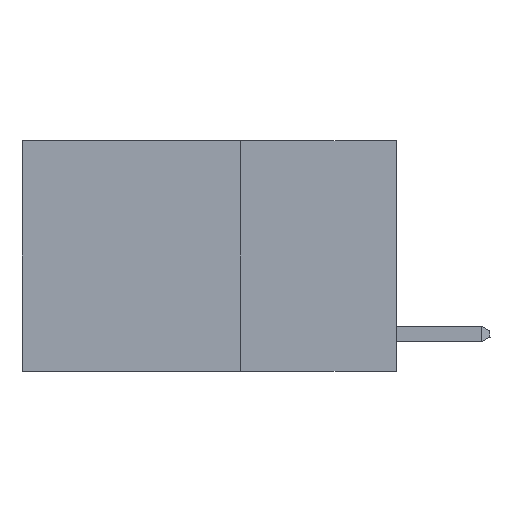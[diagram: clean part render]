
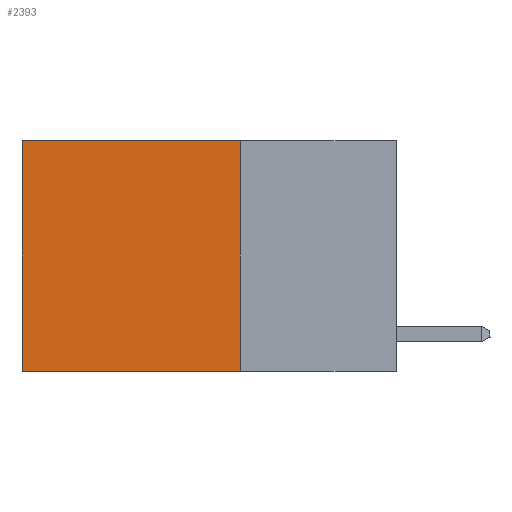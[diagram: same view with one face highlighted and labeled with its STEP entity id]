
A CAD part, left-side view. The second image highlights one B-rep face of the part: STEP entity #2393.
In plain terms, the highlighted planar face has unit normal (-1, 0, 0).
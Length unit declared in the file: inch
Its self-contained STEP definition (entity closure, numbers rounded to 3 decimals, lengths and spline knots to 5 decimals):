
#414 = EDGE_CURVE ( 'NONE', #20700, #18287, #15622, .T. ) ;
#497 = CARTESIAN_POINT ( 'NONE',  ( 0.2625, 0.25, 0. ) ) ;
#1121 = AXIS2_PLACEMENT_3D ( 'NONE', #14091, #20142, #8088 ) ;
#1443 = VERTEX_POINT ( 'NONE', #497 ) ;
#1730 = DIRECTION ( 'NONE',  ( 0., 1., 0. ) ) ;
#2393 = ADVANCED_FACE ( 'NONE', ( #16358 ), #6029, .F. ) ;
#3197 = ORIENTED_EDGE ( 'NONE', *, *, #414, .F. ) ;
#3429 = LINE ( 'NONE', #11577, #14179 ) ;
#4491 = EDGE_LOOP ( 'NONE', ( #7459, #3197, #17044, #9672 ) ) ;
#4577 = VECTOR ( 'NONE', #13738, 39.37008 ) ;
#4591 = CARTESIAN_POINT ( 'NONE',  ( 0.2625, 0.6, -0.37 ) ) ;
#6029 = PLANE ( 'NONE',  #1121 ) ;
#7459 = ORIENTED_EDGE ( 'NONE', *, *, #25188, .T. ) ;
#8088 = DIRECTION ( 'NONE',  ( 0., 0., -1. ) ) ;
#8671 = LINE ( 'NONE', #24523, #13416 ) ;
#9672 = ORIENTED_EDGE ( 'NONE', *, *, #16811, .T. ) ;
#11577 = CARTESIAN_POINT ( 'NONE',  ( 0.2625, 0.25, 0. ) ) ;
#12103 = CARTESIAN_POINT ( 'NONE',  ( 0.2625, 0.6, 0. ) ) ;
#13416 = VECTOR ( 'NONE', #14526, 39.37008 ) ;
#13738 = DIRECTION ( 'NONE',  ( 0., 0., -1. ) ) ;
#14091 = CARTESIAN_POINT ( 'NONE',  ( 0.2625, 0.25, 0. ) ) ;
#14179 = VECTOR ( 'NONE', #25609, 39.37008 ) ;
#14526 = DIRECTION ( 'NONE',  ( 0., 1., 0. ) ) ;
#15622 = LINE ( 'NONE', #21803, #20937 ) ;
#16064 = VERTEX_POINT ( 'NONE', #12103 ) ;
#16358 = FACE_OUTER_BOUND ( 'NONE', #4491, .T. ) ;
#16786 = CARTESIAN_POINT ( 'NONE',  ( 0.2625, 0.25, -0.37 ) ) ;
#16811 = EDGE_CURVE ( 'NONE', #1443, #16064, #8671, .T. ) ;
#17044 = ORIENTED_EDGE ( 'NONE', *, *, #23510, .F. ) ;
#18287 = VERTEX_POINT ( 'NONE', #4591 ) ;
#20142 = DIRECTION ( 'NONE',  ( 1., 0., 0. ) ) ;
#20700 = VERTEX_POINT ( 'NONE', #16786 ) ;
#20937 = VECTOR ( 'NONE', #1730, 39.37008 ) ;
#21803 = CARTESIAN_POINT ( 'NONE',  ( 0.2625, 0.25, -0.37 ) ) ;
#23510 = EDGE_CURVE ( 'NONE', #1443, #20700, #3429, .T. ) ;
#23750 = CARTESIAN_POINT ( 'NONE',  ( 0.2625, 0.6, 0. ) ) ;
#24523 = CARTESIAN_POINT ( 'NONE',  ( 0.2625, 0.25, 0. ) ) ;
#25188 = EDGE_CURVE ( 'NONE', #16064, #18287, #26006, .T. ) ;
#25609 = DIRECTION ( 'NONE',  ( 0., 0., -1. ) ) ;
#26006 = LINE ( 'NONE', #23750, #4577 ) ;
